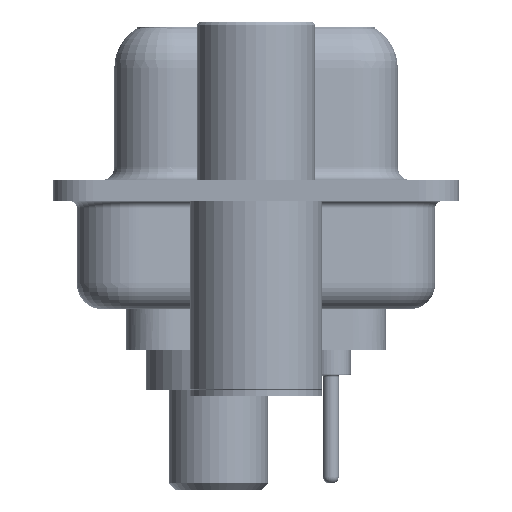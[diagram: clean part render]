
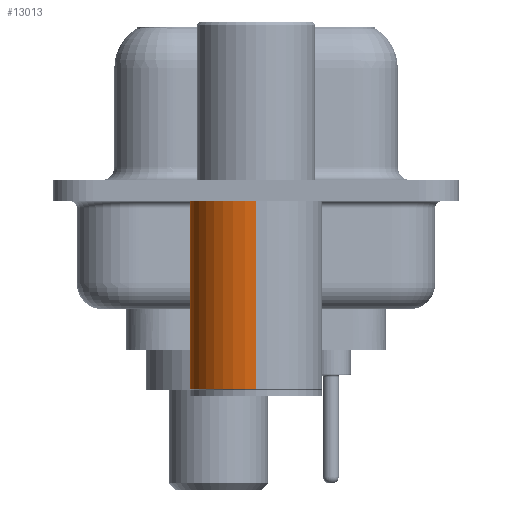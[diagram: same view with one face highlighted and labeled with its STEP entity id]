
A CAD part, left-side view. The second image highlights one B-rep face of the part: STEP entity #13013.
In plain terms, the highlighted cylindrical face has radius 2.5 mm (diameter 5 mm), a partial arc.
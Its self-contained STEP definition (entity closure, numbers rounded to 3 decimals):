
#57 = CARTESIAN_POINT ( 'NONE',  ( 2.5, 0., -7.525 ) ) ;
#1827 = DIRECTION ( 'NONE',  ( 0., 0., 1. ) ) ;
#2422 = DIRECTION ( 'NONE',  ( 1., 0., 0. ) ) ;
#3293 = DIRECTION ( 'NONE',  ( 0., 0., 1. ) ) ;
#4815 = ORIENTED_EDGE ( 'NONE', *, *, #35179, .F. ) ;
#5242 = CARTESIAN_POINT ( 'NONE',  ( 0., 0., -0.4 ) ) ;
#6336 = CIRCLE ( 'NONE', #16051, 2.5 ) ;
#6784 = VECTOR ( 'NONE', #3293, 1000. ) ;
#7013 = ORIENTED_EDGE ( 'NONE', *, *, #7047, .T. ) ;
#7047 = EDGE_CURVE ( 'NONE', #13674, #22274, #6336, .T. ) ;
#7535 = ORIENTED_EDGE ( 'NONE', *, *, #16426, .F. ) ;
#8086 = DIRECTION ( 'NONE',  ( 1., 0., 0. ) ) ;
#8852 = CARTESIAN_POINT ( 'NONE',  ( -2.5, 0., -7.525 ) ) ;
#9144 = VECTOR ( 'NONE', #36049, 1000. ) ;
#10748 = DIRECTION ( 'NONE',  ( 0., 0., 1. ) ) ;
#13013 = ADVANCED_FACE ( 'NONE', ( #31299 ), #16306, .T. ) ;
#13674 = VERTEX_POINT ( 'NONE', #57 ) ;
#16051 = AXIS2_PLACEMENT_3D ( 'NONE', #18616, #1827, #21441 ) ;
#16306 = CYLINDRICAL_SURFACE ( 'NONE', #21632, 2.5 ) ;
#16426 = EDGE_CURVE ( 'NONE', #13674, #25115, #31578, .T. ) ;
#16462 = EDGE_LOOP ( 'NONE', ( #7013, #24437, #4815, #7535 ) ) ;
#18616 = CARTESIAN_POINT ( 'NONE',  ( 0., 0., -7.525 ) ) ;
#19312 = CARTESIAN_POINT ( 'NONE',  ( 2.5, 0., 0.581 ) ) ;
#20070 = CARTESIAN_POINT ( 'NONE',  ( -2.5, 0., 0.581 ) ) ;
#21441 = DIRECTION ( 'NONE',  ( 1., 0., 0. ) ) ;
#21632 = AXIS2_PLACEMENT_3D ( 'NONE', #24521, #32874, #8086 ) ;
#22274 = VERTEX_POINT ( 'NONE', #8852 ) ;
#24437 = ORIENTED_EDGE ( 'NONE', *, *, #24611, .T. ) ;
#24521 = CARTESIAN_POINT ( 'NONE',  ( 0., 0., 0.581 ) ) ;
#24611 = EDGE_CURVE ( 'NONE', #22274, #26331, #33603, .T. ) ;
#25115 = VERTEX_POINT ( 'NONE', #33704 ) ;
#25280 = CARTESIAN_POINT ( 'NONE',  ( -2.5, 0., -0.4 ) ) ;
#26331 = VERTEX_POINT ( 'NONE', #25280 ) ;
#27923 = CIRCLE ( 'NONE', #32639, 2.5 ) ;
#31299 = FACE_OUTER_BOUND ( 'NONE', #16462, .T. ) ;
#31578 = LINE ( 'NONE', #19312, #9144 ) ;
#32639 = AXIS2_PLACEMENT_3D ( 'NONE', #5242, #10748, #2422 ) ;
#32874 = DIRECTION ( 'NONE',  ( 0., 0., 1. ) ) ;
#33603 = LINE ( 'NONE', #20070, #6784 ) ;
#33704 = CARTESIAN_POINT ( 'NONE',  ( 2.5, 0., -0.4 ) ) ;
#35179 = EDGE_CURVE ( 'NONE', #25115, #26331, #27923, .T. ) ;
#36049 = DIRECTION ( 'NONE',  ( 0., 0., 1. ) ) ;
